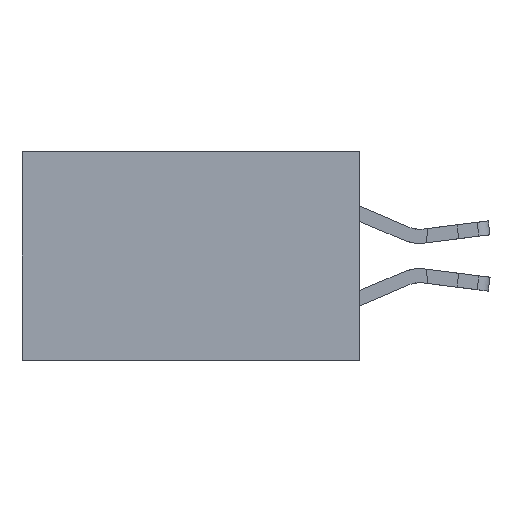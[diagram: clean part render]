
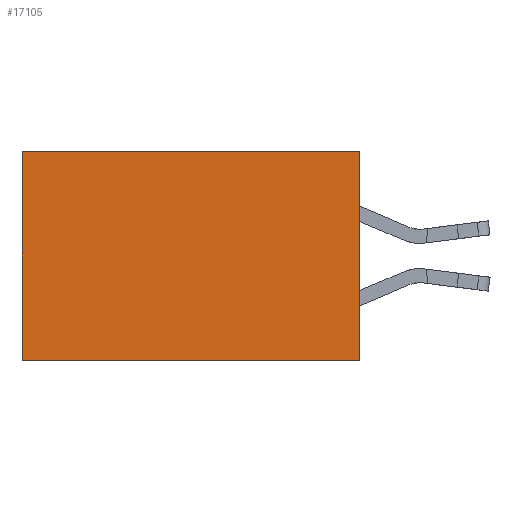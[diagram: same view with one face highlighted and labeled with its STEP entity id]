
A CAD part, left-side view. The second image highlights one B-rep face of the part: STEP entity #17105.
In plain terms, the highlighted planar face has unit normal (-1, 0, 0).
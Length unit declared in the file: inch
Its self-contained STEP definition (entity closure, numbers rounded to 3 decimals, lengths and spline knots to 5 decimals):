
#563 = EDGE_CURVE ( 'NONE', #23572, #14345, #2349, .T. ) ;
#1020 = DIRECTION ( 'NONE',  ( 0., 0., -1. ) ) ;
#1597 = VECTOR ( 'NONE', #8475, 39.37008 ) ;
#2349 = LINE ( 'NONE', #6348, #4122 ) ;
#2548 = ORIENTED_EDGE ( 'NONE', *, *, #24519, .F. ) ;
#4122 = VECTOR ( 'NONE', #16620, 39.37008 ) ;
#4158 = ORIENTED_EDGE ( 'NONE', *, *, #563, .T. ) ;
#4783 = CARTESIAN_POINT ( 'NONE',  ( 0.2875, 0., -0.37 ) ) ;
#6035 = CARTESIAN_POINT ( 'NONE',  ( 0.2875, 0.6, -0.37 ) ) ;
#6348 = CARTESIAN_POINT ( 'NONE',  ( 0.2875, 0., 0. ) ) ;
#6404 = CARTESIAN_POINT ( 'NONE',  ( 0.2875, 0., -0.37 ) ) ;
#6409 = ORIENTED_EDGE ( 'NONE', *, *, #22921, .T. ) ;
#8244 = CARTESIAN_POINT ( 'NONE',  ( 0.2875, 0., 0. ) ) ;
#8403 = DIRECTION ( 'NONE',  ( 0., 0., -1. ) ) ;
#8475 = DIRECTION ( 'NONE',  ( 0., 1., 0. ) ) ;
#9596 = EDGE_LOOP ( 'NONE', ( #6409, #20374, #2548, #4158 ) ) ;
#9908 = CARTESIAN_POINT ( 'NONE',  ( 0.2875, 0., 0. ) ) ;
#9937 = DIRECTION ( 'NONE',  ( 0., 0., -1. ) ) ;
#10572 = CARTESIAN_POINT ( 'NONE',  ( 0.2875, 0., 0. ) ) ;
#10953 = AXIS2_PLACEMENT_3D ( 'NONE', #10572, #19980, #1020 ) ;
#11159 = VECTOR ( 'NONE', #9937, 39.37008 ) ;
#11361 = LINE ( 'NONE', #6404, #1597 ) ;
#13310 = FACE_OUTER_BOUND ( 'NONE', #9596, .T. ) ;
#14194 = VERTEX_POINT ( 'NONE', #4783 ) ;
#14237 = PLANE ( 'NONE',  #10953 ) ;
#14345 = VERTEX_POINT ( 'NONE', #15910 ) ;
#15524 = CARTESIAN_POINT ( 'NONE',  ( 0.2875, 0.6, 0. ) ) ;
#15910 = CARTESIAN_POINT ( 'NONE',  ( 0.2875, 0.6, 0. ) ) ;
#16620 = DIRECTION ( 'NONE',  ( 0., 1., 0. ) ) ;
#17105 = ADVANCED_FACE ( 'NONE', ( #13310 ), #14237, .F. ) ;
#19027 = VERTEX_POINT ( 'NONE', #6035 ) ;
#19938 = LINE ( 'NONE', #8244, #21749 ) ;
#19980 = DIRECTION ( 'NONE',  ( 1., 0., 0. ) ) ;
#20374 = ORIENTED_EDGE ( 'NONE', *, *, #24555, .F. ) ;
#20624 = LINE ( 'NONE', #15524, #11159 ) ;
#21749 = VECTOR ( 'NONE', #8403, 39.37008 ) ;
#22921 = EDGE_CURVE ( 'NONE', #14345, #19027, #20624, .T. ) ;
#23572 = VERTEX_POINT ( 'NONE', #9908 ) ;
#24519 = EDGE_CURVE ( 'NONE', #23572, #14194, #19938, .T. ) ;
#24555 = EDGE_CURVE ( 'NONE', #14194, #19027, #11361, .T. ) ;
